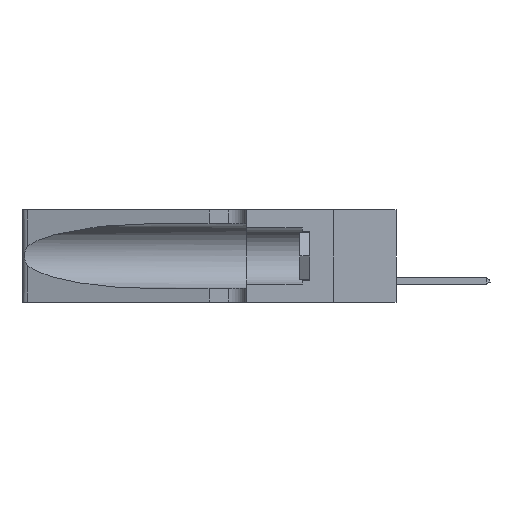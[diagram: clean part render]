
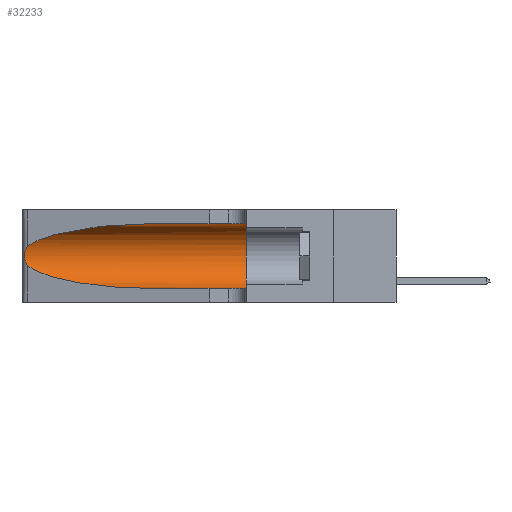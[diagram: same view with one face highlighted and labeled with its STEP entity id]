
A CAD part, left-side view. The second image highlights one B-rep face of the part: STEP entity #32233.
In plain terms, the highlighted cylindrical face has radius 3.308 mm (diameter 6.617 mm), a partial arc.
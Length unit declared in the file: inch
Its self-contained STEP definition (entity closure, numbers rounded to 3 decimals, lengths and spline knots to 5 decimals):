
#717 =( BOUNDED_CURVE ( )  B_SPLINE_CURVE ( 3, ( #15343, #15075, #33837, #37598 ),
 .UNSPECIFIED., .F., .F. ) 
 B_SPLINE_CURVE_WITH_KNOTS ( ( 4, 4 ),
 ( 3.44316, 4.71239 ),
 .UNSPECIFIED. ) 
 CURVE ( )  GEOMETRIC_REPRESENTATION_ITEM ( )  RATIONAL_B_SPLINE_CURVE ( ( 1., 0.87, 0.87, 1. ) ) 
 REPRESENTATION_ITEM ( '' )  );
#859 = DIRECTION ( 'NONE',  ( 0., -1., 0. ) ) ;
#2913 = CARTESIAN_POINT ( 'NONE',  ( 0.1305, 1.61858, 0.05475 ) ) ;
#2943 = EDGE_CURVE ( 'NONE', #4597, #31845, #40739, .T. ) ;
#3199 = LINE ( 'NONE', #31815, #41138 ) ;
#4597 = VERTEX_POINT ( 'NONE', #29619 ) ;
#5980 = DIRECTION ( 'NONE',  ( 0., -1., 0. ) ) ;
#6898 = EDGE_LOOP ( 'NONE', ( #40212, #39671, #29094, #17280, #29443, #35262 ) ) ;
#7210 = DIRECTION ( 'NONE',  ( 0., 0., 1. ) ) ;
#8258 = VERTEX_POINT ( 'NONE', #42937 ) ;
#8345 = CARTESIAN_POINT ( 'NONE',  ( 0.26018, 1.23835, 0.19895 ) ) ;
#8657 = CARTESIAN_POINT ( 'NONE',  ( 0.26075, 1.23896, 0.19203 ) ) ;
#8747 = FACE_OUTER_BOUND ( 'NONE', #6898, .T. ) ;
#10863 = CARTESIAN_POINT ( 'NONE',  ( 0.1305, 0.35, 0.31525 ) ) ;
#11760 = CARTESIAN_POINT ( 'NONE',  ( 0.25555, 1.22994, 0.2215 ) ) ;
#12416 = CARTESIAN_POINT ( 'NONE',  ( 0.1305, 0.35, 0.05475 ) ) ;
#13044 = CARTESIAN_POINT ( 'NONE',  ( 0.25487, 1.22718, 0.22369 ) ) ;
#13342 = EDGE_CURVE ( 'NONE', #8258, #25729, #14867, .T. ) ;
#14633 = EDGE_CURVE ( 'NONE', #36140, #8258, #19489, .T. ) ;
#14867 = B_SPLINE_CURVE_WITH_KNOTS ( 'NONE', 3,
 ( #31953, #11760, #35311, #42537, #28841, #8345, #8657, #32102, #28394, #21841, #35160, #35620, #15223, #15076 ),
 .UNSPECIFIED., .F., .F.,
 ( 4, 2, 2, 2, 2, 2, 4 ),
 ( 0., 0.00027, 0.00053, 0.00107, 0.0016, 0.00187, 0.00214 ),
 .UNSPECIFIED. ) ;
#15075 = CARTESIAN_POINT ( 'NONE',  ( 0.2373, 1.15595, 0.08982 ) ) ;
#15076 = CARTESIAN_POINT ( 'NONE',  ( 0.25487, 1.22718, 0.14631 ) ) ;
#15223 = CARTESIAN_POINT ( 'NONE',  ( 0.25555, 1.22993, 0.14849 ) ) ;
#15343 = CARTESIAN_POINT ( 'NONE',  ( 0.25487, 1.22718, 0.14631 ) ) ;
#17280 = ORIENTED_EDGE ( 'NONE', *, *, #2943, .T. ) ;
#18021 = VECTOR ( 'NONE', #859, 39.37008 ) ;
#19489 =( BOUNDED_CURVE ( )  B_SPLINE_CURVE ( 3, ( #43255, #19797, #26484, #13044 ),
 .UNSPECIFIED., .F., .F. ) 
 B_SPLINE_CURVE_WITH_KNOTS ( ( 4, 4 ),
 ( 1.5708, 2.84003 ),
 .UNSPECIFIED. ) 
 CURVE ( )  GEOMETRIC_REPRESENTATION_ITEM ( )  RATIONAL_B_SPLINE_CURVE ( ( 1., 0.87, 0.87, 1. ) ) 
 REPRESENTATION_ITEM ( '' )  );
#19797 = CARTESIAN_POINT ( 'NONE',  ( 0.18966, 0.96281, 0.31525 ) ) ;
#20396 = AXIS2_PLACEMENT_3D ( 'NONE', #34347, #27425, #7210 ) ;
#21841 = CARTESIAN_POINT ( 'NONE',  ( 0.25856, 1.23593, 0.16098 ) ) ;
#24467 = CYLINDRICAL_SURFACE ( 'NONE', #43512, 0.13025 ) ;
#25729 = VERTEX_POINT ( 'NONE', #42334 ) ;
#26484 = CARTESIAN_POINT ( 'NONE',  ( 0.2373, 1.15595, 0.28018 ) ) ;
#26820 = CARTESIAN_POINT ( 'NONE',  ( 0.1305, 0.72297, 0.31525 ) ) ;
#27425 = DIRECTION ( 'NONE',  ( 0., 1., 0. ) ) ;
#28394 = CARTESIAN_POINT ( 'NONE',  ( 0.26017, 1.23833, 0.17102 ) ) ;
#28841 = CARTESIAN_POINT ( 'NONE',  ( 0.25854, 1.2359, 0.20912 ) ) ;
#29094 = ORIENTED_EDGE ( 'NONE', *, *, #38251, .T. ) ;
#29443 = ORIENTED_EDGE ( 'NONE', *, *, #36900, .F. ) ;
#29619 = CARTESIAN_POINT ( 'NONE',  ( 0.1305, 0.72297, 0.05475 ) ) ;
#31815 = CARTESIAN_POINT ( 'NONE',  ( 0.1305, 1.61858, 0.31525 ) ) ;
#31845 = VERTEX_POINT ( 'NONE', #12416 ) ;
#31953 = CARTESIAN_POINT ( 'NONE',  ( 0.25487, 1.22718, 0.22369 ) ) ;
#32102 = CARTESIAN_POINT ( 'NONE',  ( 0.26075, 1.23896, 0.178 ) ) ;
#32233 = ADVANCED_FACE ( 'NONE', ( #8747 ), #24467, .F. ) ;
#33837 = CARTESIAN_POINT ( 'NONE',  ( 0.18966, 0.96281, 0.05475 ) ) ;
#34347 = CARTESIAN_POINT ( 'NONE',  ( 0.1305, 0.35, 0.185 ) ) ;
#34750 = VERTEX_POINT ( 'NONE', #10863 ) ;
#35160 = CARTESIAN_POINT ( 'NONE',  ( 0.25789, 1.23486, 0.15765 ) ) ;
#35262 = ORIENTED_EDGE ( 'NONE', *, *, #36355, .F. ) ;
#35311 = CARTESIAN_POINT ( 'NONE',  ( 0.25639, 1.23184, 0.21858 ) ) ;
#35620 = CARTESIAN_POINT ( 'NONE',  ( 0.25639, 1.23186, 0.15144 ) ) ;
#36140 = VERTEX_POINT ( 'NONE', #26820 ) ;
#36355 = EDGE_CURVE ( 'NONE', #36140, #34750, #3199, .T. ) ;
#36760 = DIRECTION ( 'NONE',  ( 0., 0., -1. ) ) ;
#36900 = EDGE_CURVE ( 'NONE', #34750, #31845, #42715, .T. ) ;
#37598 = CARTESIAN_POINT ( 'NONE',  ( 0.1305, 0.72297, 0.05475 ) ) ;
#38251 = EDGE_CURVE ( 'NONE', #25729, #4597, #717, .T. ) ;
#39671 = ORIENTED_EDGE ( 'NONE', *, *, #13342, .T. ) ;
#40212 = ORIENTED_EDGE ( 'NONE', *, *, #14633, .T. ) ;
#40739 = LINE ( 'NONE', #2913, #18021 ) ;
#41138 = VECTOR ( 'NONE', #43690, 39.37008 ) ;
#42334 = CARTESIAN_POINT ( 'NONE',  ( 0.25487, 1.22718, 0.14631 ) ) ;
#42537 = CARTESIAN_POINT ( 'NONE',  ( 0.25787, 1.23484, 0.2124 ) ) ;
#42715 = CIRCLE ( 'NONE', #20396, 0.13025 ) ;
#42937 = CARTESIAN_POINT ( 'NONE',  ( 0.25487, 1.22718, 0.22369 ) ) ;
#43079 = CARTESIAN_POINT ( 'NONE',  ( 0.1305, 1.61858, 0.185 ) ) ;
#43255 = CARTESIAN_POINT ( 'NONE',  ( 0.1305, 0.72297, 0.31525 ) ) ;
#43512 = AXIS2_PLACEMENT_3D ( 'NONE', #43079, #5980, #36760 ) ;
#43690 = DIRECTION ( 'NONE',  ( 0., -1., 0. ) ) ;
